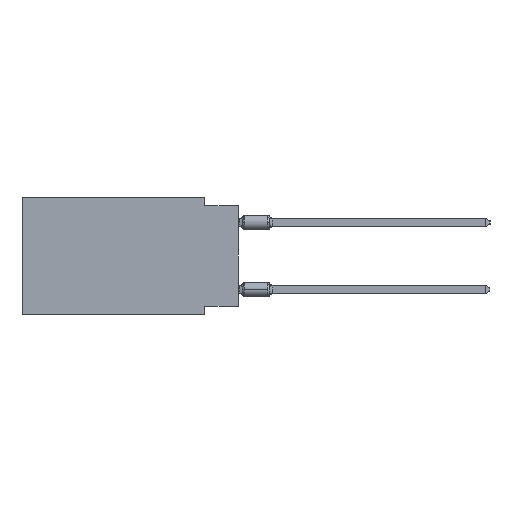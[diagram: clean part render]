
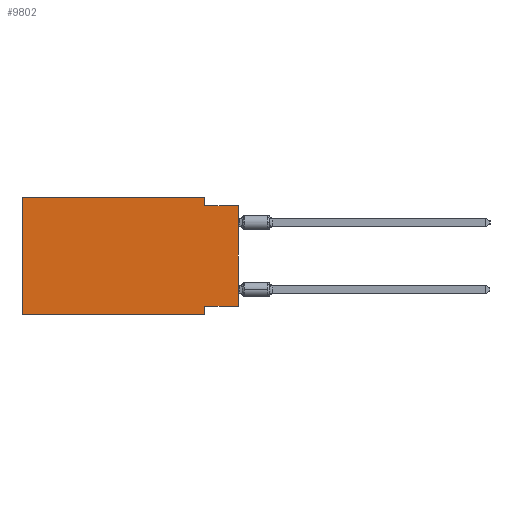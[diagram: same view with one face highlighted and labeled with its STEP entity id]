
A CAD part, left-side view. The second image highlights one B-rep face of the part: STEP entity #9802.
In plain terms, the highlighted planar face has unit normal (-1, 0, 0).
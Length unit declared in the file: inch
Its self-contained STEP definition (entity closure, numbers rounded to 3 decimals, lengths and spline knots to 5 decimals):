
#1162 = CARTESIAN_POINT ( 'NONE',  ( 0., 0.1, -0.35 ) ) ;
#1581 = CARTESIAN_POINT ( 'NONE',  ( 0., 0.1, -0.325 ) ) ;
#1708 = VERTEX_POINT ( 'NONE', #10955 ) ;
#1728 = LINE ( 'NONE', #9250, #17381 ) ;
#1862 = CARTESIAN_POINT ( 'NONE',  ( 0., 0.645, -0.35 ) ) ;
#2089 = DIRECTION ( 'NONE',  ( 0., -1., 0. ) ) ;
#2326 = CARTESIAN_POINT ( 'NONE',  ( 0., 0., -0.025 ) ) ;
#3555 = ORIENTED_EDGE ( 'NONE', *, *, #36099, .T. ) ;
#3557 = VERTEX_POINT ( 'NONE', #20598 ) ;
#5269 = DIRECTION ( 'NONE',  ( 0., -1., 0. ) ) ;
#6054 = DIRECTION ( 'NONE',  ( 0., 0., -1. ) ) ;
#6845 = ORIENTED_EDGE ( 'NONE', *, *, #37954, .F. ) ;
#8700 = LINE ( 'NONE', #19306, #29443 ) ;
#9021 = DIRECTION ( 'NONE',  ( 0., 1., 0. ) ) ;
#9250 = CARTESIAN_POINT ( 'NONE',  ( 0., 0., -0.325 ) ) ;
#9360 = VECTOR ( 'NONE', #2089, 39.37008 ) ;
#9802 = ADVANCED_FACE ( 'NONE', ( #29989 ), #42091, .F. ) ;
#10201 = LINE ( 'NONE', #37358, #25452 ) ;
#10955 = CARTESIAN_POINT ( 'NONE',  ( 0., 0., -0.325 ) ) ;
#12328 = LINE ( 'NONE', #41911, #17571 ) ;
#12596 = DIRECTION ( 'NONE',  ( 0., 0., 1. ) ) ;
#14455 = VERTEX_POINT ( 'NONE', #36483 ) ;
#14491 = ORIENTED_EDGE ( 'NONE', *, *, #21622, .F. ) ;
#16268 = VECTOR ( 'NONE', #20478, 39.37008 ) ;
#17381 = VECTOR ( 'NONE', #9021, 39.37008 ) ;
#17475 = EDGE_LOOP ( 'NONE', ( #17719, #37162, #6845, #41060, #35388, #3555, #19468, #14491 ) ) ;
#17571 = VECTOR ( 'NONE', #18965, 39.37008 ) ;
#17719 = ORIENTED_EDGE ( 'NONE', *, *, #37437, .T. ) ;
#18965 = DIRECTION ( 'NONE',  ( 0., -1., 0. ) ) ;
#19306 = CARTESIAN_POINT ( 'NONE',  ( 0., 0.1, -0.35 ) ) ;
#19468 = ORIENTED_EDGE ( 'NONE', *, *, #22081, .F. ) ;
#20096 = LINE ( 'NONE', #42839, #37364 ) ;
#20478 = DIRECTION ( 'NONE',  ( 0., 0., -1. ) ) ;
#20598 = CARTESIAN_POINT ( 'NONE',  ( 0., 0., -0.025 ) ) ;
#20946 = CARTESIAN_POINT ( 'NONE',  ( 0., 0.645, 0. ) ) ;
#21622 = EDGE_CURVE ( 'NONE', #1708, #37810, #1728, .T. ) ;
#22081 = EDGE_CURVE ( 'NONE', #37810, #28854, #8700, .T. ) ;
#24049 = AXIS2_PLACEMENT_3D ( 'NONE', #26473, #26676, #36844 ) ;
#24721 = EDGE_CURVE ( 'NONE', #27737, #28916, #25389, .T. ) ;
#25389 = LINE ( 'NONE', #38605, #40826 ) ;
#25452 = VECTOR ( 'NONE', #43129, 39.37008 ) ;
#26404 = EDGE_CURVE ( 'NONE', #31278, #27737, #20096, .T. ) ;
#26473 = CARTESIAN_POINT ( 'NONE',  ( 0., 0.645, 0. ) ) ;
#26676 = DIRECTION ( 'NONE',  ( 1., 0., 0. ) ) ;
#27737 = VERTEX_POINT ( 'NONE', #20946 ) ;
#28854 = VERTEX_POINT ( 'NONE', #1162 ) ;
#28916 = VERTEX_POINT ( 'NONE', #38927 ) ;
#29443 = VECTOR ( 'NONE', #6054, 39.37008 ) ;
#29470 = LINE ( 'NONE', #2326, #9360 ) ;
#29989 = FACE_OUTER_BOUND ( 'NONE', #17475, .T. ) ;
#30187 = LINE ( 'NONE', #37250, #16268 ) ;
#31278 = VERTEX_POINT ( 'NONE', #1862 ) ;
#35388 = ORIENTED_EDGE ( 'NONE', *, *, #26404, .F. ) ;
#36099 = EDGE_CURVE ( 'NONE', #31278, #28854, #12328, .T. ) ;
#36483 = CARTESIAN_POINT ( 'NONE',  ( 0., 0.1, -0.025 ) ) ;
#36844 = DIRECTION ( 'NONE',  ( 0., 0., -1. ) ) ;
#37162 = ORIENTED_EDGE ( 'NONE', *, *, #41079, .F. ) ;
#37250 = CARTESIAN_POINT ( 'NONE',  ( 0., 0.1, 0. ) ) ;
#37358 = CARTESIAN_POINT ( 'NONE',  ( 0., 0., 0. ) ) ;
#37364 = VECTOR ( 'NONE', #12596, 39.37008 ) ;
#37437 = EDGE_CURVE ( 'NONE', #1708, #3557, #10201, .T. ) ;
#37810 = VERTEX_POINT ( 'NONE', #1581 ) ;
#37954 = EDGE_CURVE ( 'NONE', #28916, #14455, #30187, .T. ) ;
#38605 = CARTESIAN_POINT ( 'NONE',  ( 0., 0.645, 0. ) ) ;
#38927 = CARTESIAN_POINT ( 'NONE',  ( 0., 0.1, 0. ) ) ;
#40826 = VECTOR ( 'NONE', #5269, 39.37008 ) ;
#41060 = ORIENTED_EDGE ( 'NONE', *, *, #24721, .F. ) ;
#41079 = EDGE_CURVE ( 'NONE', #14455, #3557, #29470, .T. ) ;
#41911 = CARTESIAN_POINT ( 'NONE',  ( 0., 0.645, -0.35 ) ) ;
#42091 = PLANE ( 'NONE',  #24049 ) ;
#42839 = CARTESIAN_POINT ( 'NONE',  ( 0., 0.645, 0. ) ) ;
#43129 = DIRECTION ( 'NONE',  ( 0., 0., 1. ) ) ;
